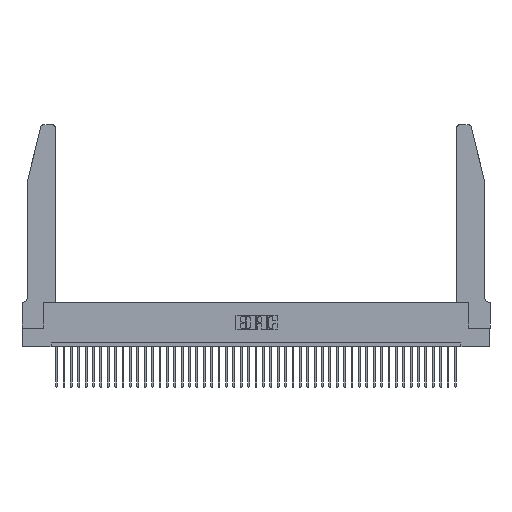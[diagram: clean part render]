
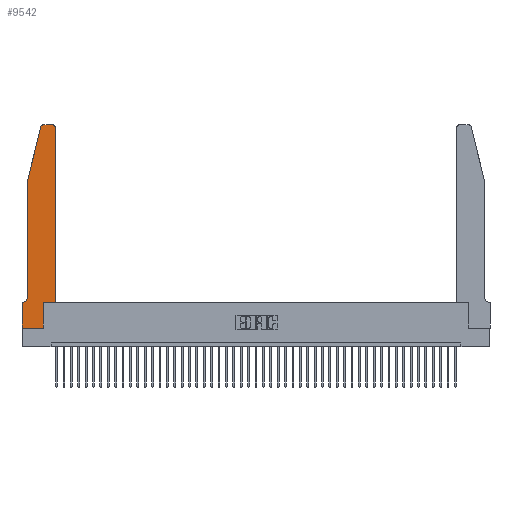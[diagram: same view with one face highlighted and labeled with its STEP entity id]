
A CAD part, top view. The second image highlights one B-rep face of the part: STEP entity #9542.
In plain terms, the highlighted planar face has unit normal (0, 0, 1).
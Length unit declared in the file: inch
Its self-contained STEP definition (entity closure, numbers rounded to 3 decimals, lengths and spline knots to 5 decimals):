
#920 = LINE ( 'NONE', #20059, #25655 ) ;
#1596 = EDGE_CURVE ( 'NONE', #18830, #26450, #920, .T. ) ;
#1948 = VERTEX_POINT ( 'NONE', #43441 ) ;
#1953 = CARTESIAN_POINT ( 'NONE',  ( 0.284, 2.75, 0.37 ) ) ;
#2623 = ORIENTED_EDGE ( 'NONE', *, *, #25779, .T. ) ;
#2886 = EDGE_CURVE ( 'NONE', #14310, #40325, #42655, .T. ) ;
#3155 = VECTOR ( 'NONE', #16267, 39.37008 ) ;
#3292 = DIRECTION ( 'NONE',  ( -1., 0., 0. ) ) ;
#3800 = CIRCLE ( 'NONE', #39020, 0.07 ) ;
#3854 = CARTESIAN_POINT ( 'NONE',  ( 0.4505, 0.35, 0.37 ) ) ;
#3856 = DIRECTION ( 'NONE',  ( 0., 1., 0. ) ) ;
#3864 = DIRECTION ( 'NONE',  ( 0., 1., 0. ) ) ;
#4199 = DIRECTION ( 'NONE',  ( 0., 0., 1. ) ) ;
#4260 = AXIS2_PLACEMENT_3D ( 'NONE', #24353, #34431, #41010 ) ;
#4353 = DIRECTION ( 'NONE',  ( 1., 0., 0. ) ) ;
#4461 = EDGE_CURVE ( 'NONE', #1948, #18385, #26974, .T. ) ;
#4561 = LINE ( 'NONE', #21837, #14760 ) ;
#5421 = DIRECTION ( 'NONE',  ( 0., 0., -1. ) ) ;
#5967 = CARTESIAN_POINT ( 'NONE',  ( 0.2605, 2.75, 0.37 ) ) ;
#6494 = CARTESIAN_POINT ( 'NONE',  ( 0.4505, 0.35, 0.37 ) ) ;
#9478 = ORIENTED_EDGE ( 'NONE', *, *, #20260, .T. ) ;
#9542 = ADVANCED_FACE ( 'NONE', ( #36831 ), #31937, .T. ) ;
#10130 = LINE ( 'NONE', #5967, #3155 ) ;
#11166 = ORIENTED_EDGE ( 'NONE', *, *, #4461, .T. ) ;
#11402 = DIRECTION ( 'NONE',  ( 0., 0., 1. ) ) ;
#11408 = CARTESIAN_POINT ( 'NONE',  ( 0., 0.35, 0.37 ) ) ;
#12451 = CARTESIAN_POINT ( 'NONE',  ( 0.0055, 0.42, 0.37 ) ) ;
#12913 = VERTEX_POINT ( 'NONE', #23080 ) ;
#13171 = VERTEX_POINT ( 'NONE', #32837 ) ;
#13730 = CIRCLE ( 'NONE', #4260, 0.03 ) ;
#14098 = CARTESIAN_POINT ( 'NONE',  ( 0.0755, 2., 0.37 ) ) ;
#14191 = EDGE_LOOP ( 'NONE', ( #15949, #24574, #43812, #11166, #9478, #42676, #2623, #33329, #40178, #26823, #17586, #21725 ) ) ;
#14263 = DIRECTION ( 'NONE',  ( 1., 0., 0. ) ) ;
#14310 = VERTEX_POINT ( 'NONE', #16155 ) ;
#14760 = VECTOR ( 'NONE', #3856, 39.37008 ) ;
#15103 = CARTESIAN_POINT ( 'NONE',  ( 0.4505, 0.35, 0.37 ) ) ;
#15348 = DIRECTION ( 'NONE',  ( 0., -1., 0. ) ) ;
#15949 = ORIENTED_EDGE ( 'NONE', *, *, #39064, .T. ) ;
#16155 = CARTESIAN_POINT ( 'NONE',  ( 0., 0., 0.37 ) ) ;
#16267 = DIRECTION ( 'NONE',  ( -1., 0., 0. ) ) ;
#17586 = ORIENTED_EDGE ( 'NONE', *, *, #28836, .T. ) ;
#17660 = LINE ( 'NONE', #43666, #37038 ) ;
#17770 = CARTESIAN_POINT ( 'NONE',  ( 0.0755, 0.42, 0.37 ) ) ;
#18385 = VERTEX_POINT ( 'NONE', #17770 ) ;
#18521 = DIRECTION ( 'NONE',  ( 1., 0., 0. ) ) ;
#18830 = VERTEX_POINT ( 'NONE', #30460 ) ;
#20059 = CARTESIAN_POINT ( 'NONE',  ( 0.0755, 0.35, 0.37 ) ) ;
#20260 = EDGE_CURVE ( 'NONE', #18385, #18830, #3800, .T. ) ;
#21009 = VECTOR ( 'NONE', #15348, 39.37008 ) ;
#21725 = ORIENTED_EDGE ( 'NONE', *, *, #40464, .T. ) ;
#21773 = AXIS2_PLACEMENT_3D ( 'NONE', #25035, #11402, #14263 ) ;
#21837 = CARTESIAN_POINT ( 'NONE',  ( 0.2865, 0.35, 0.37 ) ) ;
#23080 = CARTESIAN_POINT ( 'NONE',  ( 0.2865, 0.35, 0.37 ) ) ;
#23240 = CARTESIAN_POINT ( 'NONE',  ( 0., 0., 0.37 ) ) ;
#23300 = CIRCLE ( 'NONE', #21773, 0.03 ) ;
#24353 = CARTESIAN_POINT ( 'NONE',  ( 0.4205, 2.72, 0.37 ) ) ;
#24388 = DIRECTION ( 'NONE',  ( 1., 0., 0. ) ) ;
#24574 = ORIENTED_EDGE ( 'NONE', *, *, #28771, .T. ) ;
#25035 = CARTESIAN_POINT ( 'NONE',  ( 0.284, 2.72, 0.37 ) ) ;
#25053 = VECTOR ( 'NONE', #41208, 39.37008 ) ;
#25655 = VECTOR ( 'NONE', #3292, 39.37008 ) ;
#25779 = EDGE_CURVE ( 'NONE', #26450, #14310, #17660, .T. ) ;
#26450 = VERTEX_POINT ( 'NONE', #39235 ) ;
#26823 = ORIENTED_EDGE ( 'NONE', *, *, #42023, .T. ) ;
#26974 = LINE ( 'NONE', #42121, #21009 ) ;
#27548 = VERTEX_POINT ( 'NONE', #39319 ) ;
#28140 = EDGE_CURVE ( 'NONE', #40325, #12913, #4561, .T. ) ;
#28771 = EDGE_CURVE ( 'NONE', #43893, #13171, #23300, .T. ) ;
#28836 = EDGE_CURVE ( 'NONE', #31270, #27548, #31869, .T. ) ;
#29271 = VECTOR ( 'NONE', #24388, 39.37008 ) ;
#29396 = DIRECTION ( 'NONE',  ( -1., 0., 0. ) ) ;
#29759 = DIRECTION ( 'NONE',  ( 0., -1., 0. ) ) ;
#29778 = VECTOR ( 'NONE', #3864, 39.37008 ) ;
#30460 = CARTESIAN_POINT ( 'NONE',  ( 0.0055, 0.35, 0.37 ) ) ;
#31270 = VERTEX_POINT ( 'NONE', #3854 ) ;
#31275 = VECTOR ( 'NONE', #18521, 39.37008 ) ;
#31869 = LINE ( 'NONE', #6494, #29778 ) ;
#31937 = PLANE ( 'NONE',  #37108 ) ;
#32837 = CARTESIAN_POINT ( 'NONE',  ( 0.25487, 2.72718, 0.37 ) ) ;
#32865 = VERTEX_POINT ( 'NONE', #38124 ) ;
#33329 = ORIENTED_EDGE ( 'NONE', *, *, #2886, .T. ) ;
#34431 = DIRECTION ( 'NONE',  ( 0., 0., 1. ) ) ;
#35497 = EDGE_CURVE ( 'NONE', #13171, #1948, #38451, .T. ) ;
#36831 = FACE_OUTER_BOUND ( 'NONE', #14191, .T. ) ;
#37038 = VECTOR ( 'NONE', #29759, 39.37008 ) ;
#37108 = AXIS2_PLACEMENT_3D ( 'NONE', #11408, #4199, #4353 ) ;
#38124 = CARTESIAN_POINT ( 'NONE',  ( 0.4205, 2.75, 0.37 ) ) ;
#38451 = LINE ( 'NONE', #14098, #25053 ) ;
#39020 = AXIS2_PLACEMENT_3D ( 'NONE', #12451, #5421, #29396 ) ;
#39064 = EDGE_CURVE ( 'NONE', #32865, #43893, #10130, .T. ) ;
#39235 = CARTESIAN_POINT ( 'NONE',  ( 0., 0.35, 0.37 ) ) ;
#39319 = CARTESIAN_POINT ( 'NONE',  ( 0.4505, 2.72, 0.37 ) ) ;
#39393 = CARTESIAN_POINT ( 'NONE',  ( 0.2865, 0., 0.37 ) ) ;
#40178 = ORIENTED_EDGE ( 'NONE', *, *, #28140, .T. ) ;
#40325 = VERTEX_POINT ( 'NONE', #39393 ) ;
#40428 = LINE ( 'NONE', #15103, #31275 ) ;
#40464 = EDGE_CURVE ( 'NONE', #27548, #32865, #13730, .T. ) ;
#41010 = DIRECTION ( 'NONE',  ( 1., 0., 0. ) ) ;
#41208 = DIRECTION ( 'NONE',  ( -0.239, -0.971, 0. ) ) ;
#42023 = EDGE_CURVE ( 'NONE', #12913, #31270, #40428, .T. ) ;
#42121 = CARTESIAN_POINT ( 'NONE',  ( 0.0755, 2., 0.37 ) ) ;
#42655 = LINE ( 'NONE', #23240, #29271 ) ;
#42676 = ORIENTED_EDGE ( 'NONE', *, *, #1596, .T. ) ;
#43441 = CARTESIAN_POINT ( 'NONE',  ( 0.0755, 2., 0.37 ) ) ;
#43666 = CARTESIAN_POINT ( 'NONE',  ( 0., 0., 0.37 ) ) ;
#43812 = ORIENTED_EDGE ( 'NONE', *, *, #35497, .T. ) ;
#43893 = VERTEX_POINT ( 'NONE', #1953 ) ;
